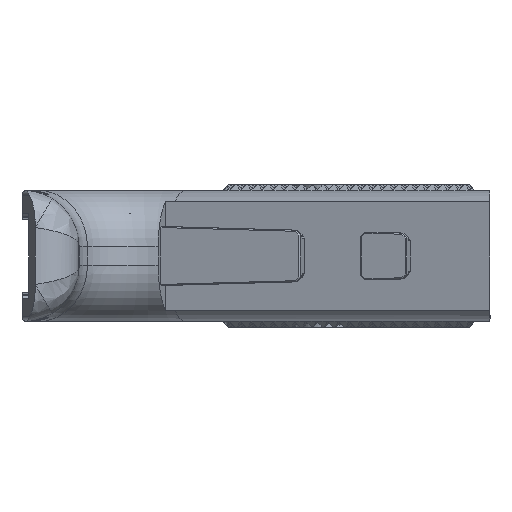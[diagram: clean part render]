
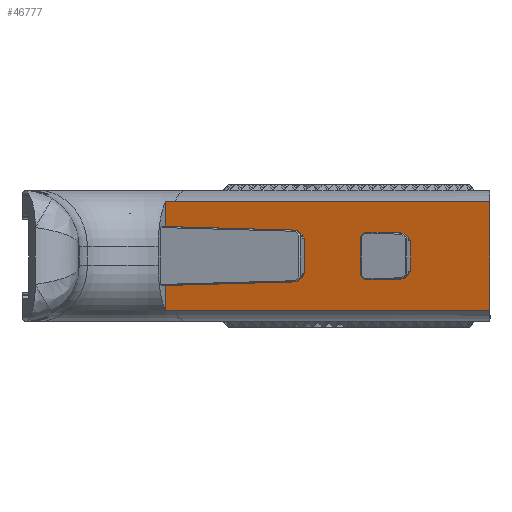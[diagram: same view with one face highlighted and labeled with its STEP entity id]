
A CAD part, left-side view. The second image highlights one B-rep face of the part: STEP entity #46777.
In plain terms, the highlighted planar face has unit normal (-0.951, 0.309, 0).
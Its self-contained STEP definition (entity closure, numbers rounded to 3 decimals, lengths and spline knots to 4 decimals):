
#54=FACE_BOUND('',#8969,.T.);
#3125=PLANE('',#49864);
#5958=FACE_OUTER_BOUND('',#8968,.T.);
#8968=EDGE_LOOP('',(#41861,#41862,#41863,#41864,#41865,#41866,#41867,#41868,
#41869,#41870,#41871,#41872));
#8969=EDGE_LOOP('',(#41873,#41874,#41875,#41876,#41877,#41878,#41879,#41880,
#41881));
#14212=LINE('',#89619,#19799);
#14230=LINE('',#89657,#19817);
#14238=LINE('',#89674,#19825);
#14243=LINE('',#89683,#19830);
#14245=LINE('',#89686,#19832);
#14247=LINE('',#89691,#19834);
#14249=LINE('',#89695,#19836);
#14251=LINE('',#89698,#19838);
#14253=LINE('',#89702,#19840);
#14254=LINE('',#89704,#19841);
#14260=LINE('',#89717,#19847);
#14262=LINE('',#89721,#19849);
#14263=LINE('',#89724,#19850);
#14265=LINE('',#89728,#19852);
#14266=LINE('',#89738,#19853);
#14267=LINE('',#89740,#19854);
#14268=LINE('',#89742,#19855);
#14269=LINE('',#89752,#19856);
#14270=LINE('',#89753,#19857);
#19799=VECTOR('',#60585,0.3937);
#19817=VECTOR('',#60621,0.3937);
#19825=VECTOR('',#60635,0.3937);
#19830=VECTOR('',#60644,0.3937);
#19832=VECTOR('',#60648,0.3937);
#19834=VECTOR('',#60652,0.3937);
#19836=VECTOR('',#60656,0.3937);
#19838=VECTOR('',#60660,0.3937);
#19840=VECTOR('',#60664,0.3937);
#19841=VECTOR('',#60667,0.3937);
#19847=VECTOR('',#60683,0.3937);
#19849=VECTOR('',#60687,0.3937);
#19850=VECTOR('',#60690,0.3937);
#19852=VECTOR('',#60694,0.3937);
#19853=VECTOR('',#60695,0.3937);
#19854=VECTOR('',#60696,0.3937);
#19855=VECTOR('',#60697,0.3937);
#19856=VECTOR('',#60698,0.3937);
#19857=VECTOR('',#60699,0.3937);
#20945=B_SPLINE_CURVE_WITH_KNOTS('',3,(#89730,#89731,#89732,#89733,#89734,
#89735,#89736),.UNSPECIFIED.,.F.,.F.,(4,3,4),(0.,0.1181,0.2155),
 .UNSPECIFIED.);
#20946=B_SPLINE_CURVE_WITH_KNOTS('',3,(#89744,#89745,#89746,#89747,#89748,
#89749,#89750),.UNSPECIFIED.,.F.,.F.,(4,3,4),(-0.2155,-0.1181,
0.),.UNSPECIFIED.);
#23885=VERTEX_POINT('',#89616);
#23886=VERTEX_POINT('',#89618);
#23896=VERTEX_POINT('',#89654);
#23897=VERTEX_POINT('',#89656);
#23902=VERTEX_POINT('',#89671);
#23903=VERTEX_POINT('',#89673);
#23905=VERTEX_POINT('',#89682);
#23906=VERTEX_POINT('',#89688);
#23907=VERTEX_POINT('',#89690);
#23908=VERTEX_POINT('',#89694);
#23909=VERTEX_POINT('',#89700);
#23911=VERTEX_POINT('',#89715);
#23912=VERTEX_POINT('',#89719);
#23913=VERTEX_POINT('',#89723);
#23914=VERTEX_POINT('',#89727);
#23915=VERTEX_POINT('',#89729);
#23916=VERTEX_POINT('',#89737);
#23917=VERTEX_POINT('',#89739);
#23918=VERTEX_POINT('',#89741);
#23919=VERTEX_POINT('',#89743);
#23920=VERTEX_POINT('',#89751);
#29973=EDGE_CURVE('',#23886,#23885,#14212,.T.);
#29991=EDGE_CURVE('',#23896,#23897,#14230,.T.);
#29999=EDGE_CURVE('',#23902,#23903,#14238,.F.);
#30004=EDGE_CURVE('',#23886,#23905,#14243,.F.);
#30006=EDGE_CURVE('',#23902,#23905,#14245,.T.);
#30008=EDGE_CURVE('',#23906,#23907,#14247,.F.);
#30010=EDGE_CURVE('',#23908,#23907,#14249,.T.);
#30012=EDGE_CURVE('',#23906,#23903,#14251,.T.);
#30014=EDGE_CURVE('',#23909,#23885,#14253,.F.);
#30015=EDGE_CURVE('',#23908,#23909,#14254,.F.);
#30021=EDGE_CURVE('',#23911,#23896,#14260,.F.);
#30023=EDGE_CURVE('',#23911,#23912,#14262,.T.);
#30024=EDGE_CURVE('',#23897,#23913,#14263,.F.);
#30026=EDGE_CURVE('',#23914,#23912,#14265,.T.);
#30027=EDGE_CURVE('',#23915,#23914,#20945,.T.);
#30028=EDGE_CURVE('',#23916,#23915,#14266,.T.);
#30029=EDGE_CURVE('',#23917,#23916,#14267,.T.);
#30030=EDGE_CURVE('',#23918,#23917,#14268,.T.);
#30031=EDGE_CURVE('',#23919,#23918,#20946,.T.);
#30032=EDGE_CURVE('',#23920,#23919,#14269,.T.);
#30033=EDGE_CURVE('',#23920,#23913,#14270,.T.);
#41861=ORIENTED_EDGE('',*,*,#30023,.T.);
#41862=ORIENTED_EDGE('',*,*,#30026,.F.);
#41863=ORIENTED_EDGE('',*,*,#30027,.F.);
#41864=ORIENTED_EDGE('',*,*,#30028,.F.);
#41865=ORIENTED_EDGE('',*,*,#30029,.F.);
#41866=ORIENTED_EDGE('',*,*,#30030,.F.);
#41867=ORIENTED_EDGE('',*,*,#30031,.F.);
#41868=ORIENTED_EDGE('',*,*,#30032,.F.);
#41869=ORIENTED_EDGE('',*,*,#30033,.T.);
#41870=ORIENTED_EDGE('',*,*,#30024,.F.);
#41871=ORIENTED_EDGE('',*,*,#29991,.F.);
#41872=ORIENTED_EDGE('',*,*,#30021,.F.);
#41873=ORIENTED_EDGE('',*,*,#29973,.T.);
#41874=ORIENTED_EDGE('',*,*,#30014,.F.);
#41875=ORIENTED_EDGE('',*,*,#30015,.F.);
#41876=ORIENTED_EDGE('',*,*,#30010,.T.);
#41877=ORIENTED_EDGE('',*,*,#30008,.F.);
#41878=ORIENTED_EDGE('',*,*,#30012,.T.);
#41879=ORIENTED_EDGE('',*,*,#29999,.F.);
#41880=ORIENTED_EDGE('',*,*,#30006,.T.);
#41881=ORIENTED_EDGE('',*,*,#30004,.F.);
#46777=ADVANCED_FACE('',(#5958,#54),#3125,.T.);
#49864=AXIS2_PLACEMENT_3D('',#89726,#60692,#60693);
#60585=DIRECTION('',(0.,0.,1.));
#60621=DIRECTION('',(0.,0.,1.));
#60635=DIRECTION('',(0.216,0.664,-0.716));
#60644=DIRECTION('',(0.221,0.681,0.698));
#60648=DIRECTION('',(0.309,0.951,-0.026));
#60652=DIRECTION('',(-0.216,-0.664,-0.716));
#60656=DIRECTION('',(-0.309,-0.951,-0.026));
#60660=DIRECTION('',(0.,0.,-1.));
#60664=DIRECTION('',(-0.12,-0.37,0.921));
#60667=DIRECTION('',(-0.221,-0.681,0.698));
#60683=DIRECTION('',(0.216,0.664,-0.716));
#60687=DIRECTION('',(0.309,0.951,-0.026));
#60690=DIRECTION('',(-0.216,-0.664,-0.716));
#60692=DIRECTION('center_axis',(-0.951,0.309,0.));
#60693=DIRECTION('ref_axis',(0.,0.,
1.));
#60694=DIRECTION('',(0.,0.,1.));
#60695=DIRECTION('',(0.309,0.951,0.));
#60696=DIRECTION('',(0.,0.,-1.));
#60697=DIRECTION('',(-0.309,-0.951,0.));
#60698=DIRECTION('',(0.,0.,1.));
#60699=DIRECTION('',(-0.309,-0.951,-0.026));
#89616=CARTESIAN_POINT('',(-2.8962,-0.8838,-0.6352));
#89618=CARTESIAN_POINT('',(-2.8962,-0.8838,-0.9101));
#89619=CARTESIAN_POINT('',(-2.8962,-0.8838,-0.7677));
#89654=CARTESIAN_POINT('',(-2.7262,-0.3607,-0.9245));
#89656=CARTESIAN_POINT('',(-2.7262,-0.3607,-0.6109));
#89657=CARTESIAN_POINT('',(-2.7262,-0.3607,-0.9154));
#89671=CARTESIAN_POINT('',(-3.0247,-1.2792,-0.909));
#89673=CARTESIAN_POINT('',(-3.0277,-1.2886,-0.8989));
#89674=CARTESIAN_POINT('',(-2.9908,-1.1749,-1.0217));
#89682=CARTESIAN_POINT('',(-2.8992,-0.8932,-0.9197));
#89683=CARTESIAN_POINT('',(-2.8709,-0.806,-0.8303));
#89686=CARTESIAN_POINT('',(-3.0469,-1.3476,-0.9072));
#89688=CARTESIAN_POINT('',(-3.0277,-1.2886,-0.6365));
#89690=CARTESIAN_POINT('',(-3.0247,-1.2792,-0.6264));
#89691=CARTESIAN_POINT('',(-2.9908,-1.1749,-0.5138));
#89694=CARTESIAN_POINT('',(-2.8992,-0.8932,-0.6158));
#89695=CARTESIAN_POINT('',(-3.0469,-1.3476,-0.6283));
#89698=CARTESIAN_POINT('',(-3.0277,-1.2886,-0.899));
#89700=CARTESIAN_POINT('',(-2.8984,-0.8905,-0.6185));
#89702=CARTESIAN_POINT('',(-2.885,-0.8493,-0.7213));
#89704=CARTESIAN_POINT('',(-2.8709,-0.806,-0.7051));
#89715=CARTESIAN_POINT('',(-2.7232,-0.3514,-0.9346));
#89717=CARTESIAN_POINT('',(-2.7647,-0.479,-0.7968));
#89719=CARTESIAN_POINT('',(-2.3324,0.8513,-0.9677));
#89721=CARTESIAN_POINT('',(-3.0469,-1.3476,-0.9072));
#89723=CARTESIAN_POINT('',(-2.7232,-0.3514,-0.6008));
#89724=CARTESIAN_POINT('',(-2.7647,-0.479,-0.7386));
#89726=CARTESIAN_POINT('Origin',(-2.8375,-0.7031,-0.7677));
#89727=CARTESIAN_POINT('',(-2.3324,0.8513,-1.2459));
#89728=CARTESIAN_POINT('',(-2.3324,0.8513,-1.0302));
#89729=CARTESIAN_POINT('',(-2.3592,0.7689,-1.2425));
#89730=CARTESIAN_POINT('Ctrl Pts',(-2.3592,0.7689,
-1.2425));
#89731=CARTESIAN_POINT('Ctrl Pts',(-2.3544,0.7836,
-1.2425));
#89732=CARTESIAN_POINT('Ctrl Pts',(-2.3495,0.7986,
-1.2428));
#89733=CARTESIAN_POINT('Ctrl Pts',(-2.3446,0.8138,
-1.2435));
#89734=CARTESIAN_POINT('Ctrl Pts',(-2.3405,0.8264,
-1.2441));
#89735=CARTESIAN_POINT('Ctrl Pts',(-2.3365,0.8388,
-1.2449));
#89736=CARTESIAN_POINT('Ctrl Pts',(-2.3324,0.8513,-1.2459));
#89737=CARTESIAN_POINT('',(-3.2516,-1.9775,-1.2425));
#89738=CARTESIAN_POINT('',(-2.1969,1.2684,-1.2425));
#89739=CARTESIAN_POINT('',(-3.2516,-1.9775,-0.2929));
#89740=CARTESIAN_POINT('',(-3.2516,-1.9775,-0.3839));
#89741=CARTESIAN_POINT('',(-2.3592,0.7689,-0.2929));
#89742=CARTESIAN_POINT('',(-2.6906,-0.2509,-0.2929));
#89743=CARTESIAN_POINT('',(-2.3324,0.8513,-0.2895));
#89744=CARTESIAN_POINT('Ctrl Pts',(-2.3324,0.8513,-0.2895));
#89745=CARTESIAN_POINT('Ctrl Pts',(-2.3365,0.8388,
-0.2905));
#89746=CARTESIAN_POINT('Ctrl Pts',(-2.3405,0.8264,
-0.2913));
#89747=CARTESIAN_POINT('Ctrl Pts',(-2.3446,0.8138,
-0.2919));
#89748=CARTESIAN_POINT('Ctrl Pts',(-2.3495,0.7986,
-0.2926));
#89749=CARTESIAN_POINT('Ctrl Pts',(-2.3544,0.7836,
-0.2929));
#89750=CARTESIAN_POINT('Ctrl Pts',(-2.3592,0.7689,
-0.2929));
#89751=CARTESIAN_POINT('',(-2.3324,0.8513,-0.5677));
#89752=CARTESIAN_POINT('',(-2.3324,0.8513,-0.7677));
#89753=CARTESIAN_POINT('',(-3.0469,-1.3476,-0.6283));
